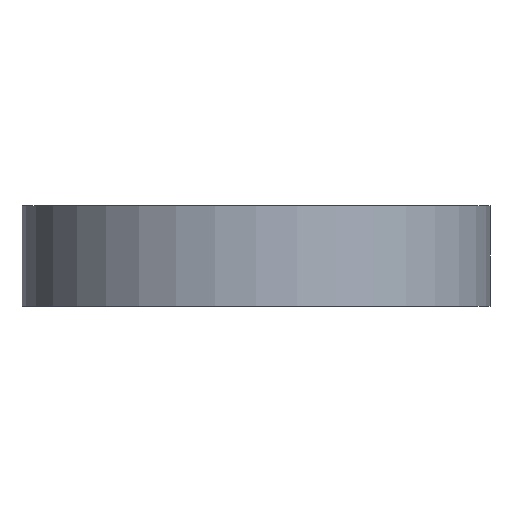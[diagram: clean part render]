
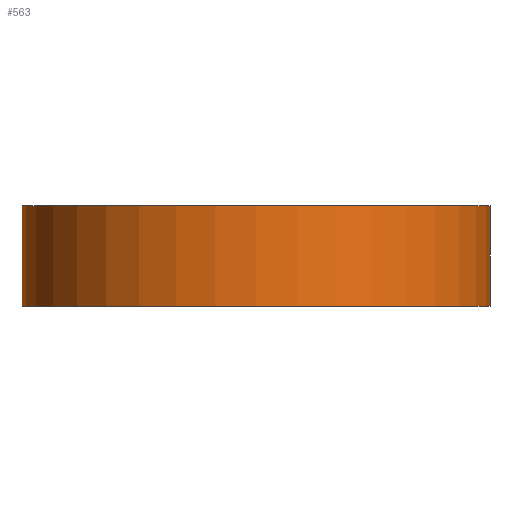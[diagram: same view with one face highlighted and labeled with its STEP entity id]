
A CAD part, front view. The second image highlights one B-rep face of the part: STEP entity #563.
In plain terms, the highlighted cylindrical face has radius 18.542 mm (diameter 37.084 mm), a full revolution.
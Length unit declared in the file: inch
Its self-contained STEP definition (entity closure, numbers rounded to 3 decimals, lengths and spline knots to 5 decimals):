
#7 = AXIS2_PLACEMENT_3D ( 'NONE', #976, #507, #44 ) ;
#44 = DIRECTION ( 'NONE',  ( 1., 0., 0. ) ) ;
#58 = AXIS2_PLACEMENT_3D ( 'NONE', #272, #818, #347 ) ;
#112 = AXIS2_PLACEMENT_3D ( 'NONE', #254, #268, #738 ) ;
#162 = CYLINDRICAL_SURFACE ( 'NONE', #112, 0.73 ) ;
#254 = CARTESIAN_POINT ( 'NONE',  ( 0., 0., 0.315 ) ) ;
#268 = DIRECTION ( 'NONE',  ( 0., 0., -1. ) ) ;
#272 = CARTESIAN_POINT ( 'NONE',  ( 0., 0., 0.315 ) ) ;
#329 = ORIENTED_EDGE ( 'NONE', *, *, #622, .T. ) ;
#347 = DIRECTION ( 'NONE',  ( 1., 0., 0. ) ) ;
#365 = CIRCLE ( 'NONE', #58, 0.73 ) ;
#379 = VERTEX_POINT ( 'NONE', #816 ) ;
#394 = FACE_OUTER_BOUND ( 'NONE', #930, .T. ) ;
#424 = CARTESIAN_POINT ( 'NONE',  ( 0.73, 0., 0.315 ) ) ;
#507 = DIRECTION ( 'NONE',  ( 0., 0., 1. ) ) ;
#563 = ADVANCED_FACE ( 'NONE', ( #810, #394 ), #162, .T. ) ;
#568 = EDGE_CURVE ( 'NONE', #588, #588, #365, .T. ) ;
#588 = VERTEX_POINT ( 'NONE', #424 ) ;
#622 = EDGE_CURVE ( 'NONE', #379, #379, #787, .T. ) ;
#738 = DIRECTION ( 'NONE',  ( -1., 0., 0. ) ) ;
#787 = CIRCLE ( 'NONE', #7, 0.73 ) ;
#810 = FACE_OUTER_BOUND ( 'NONE', #850, .T. ) ;
#816 = CARTESIAN_POINT ( 'NONE',  ( 0.73, 0., 0. ) ) ;
#818 = DIRECTION ( 'NONE',  ( 0., 0., 1. ) ) ;
#850 = EDGE_LOOP ( 'NONE', ( #1007 ) ) ;
#930 = EDGE_LOOP ( 'NONE', ( #329 ) ) ;
#976 = CARTESIAN_POINT ( 'NONE',  ( 0., 0., 0. ) ) ;
#1007 = ORIENTED_EDGE ( 'NONE', *, *, #568, .F. ) ;
